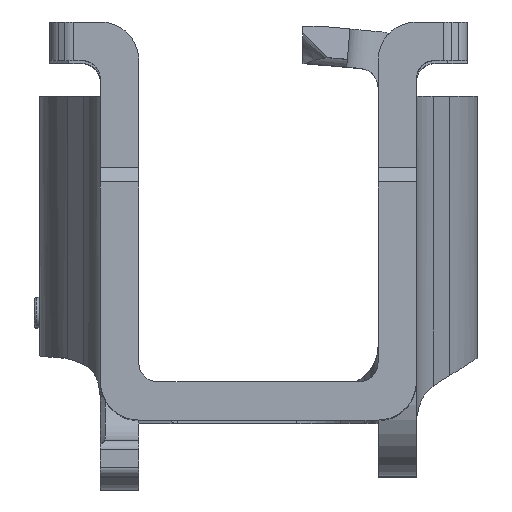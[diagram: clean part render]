
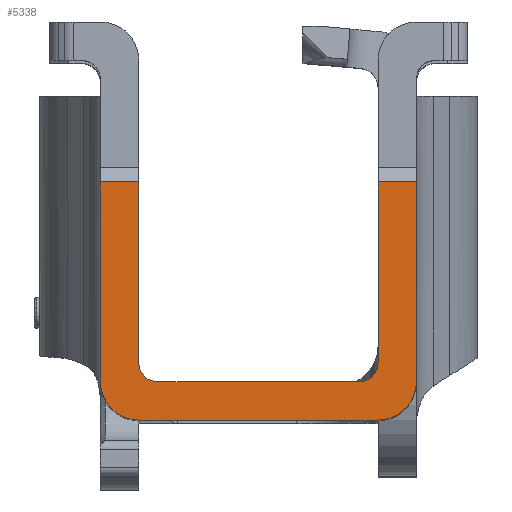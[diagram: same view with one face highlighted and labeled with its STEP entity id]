
A CAD part, top view. The second image highlights one B-rep face of the part: STEP entity #5338.
In plain terms, the highlighted planar face has unit normal (0, 0, 1).
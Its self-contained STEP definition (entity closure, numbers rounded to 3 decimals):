
#235=PLANE('',#5881);
#502=FACE_OUTER_BOUND('',#802,.T.);
#802=EDGE_LOOP('',(#4935,#4936,#4937,#4938,#4939,#4940,#4941,#4942,#4943,
#4944,#4945,#4946));
#888=LINE('',#7627,#1386);
#1201=LINE('',#8884,#1699);
#1208=LINE('',#8909,#1706);
#1216=LINE('',#8926,#1714);
#1217=LINE('',#8929,#1715);
#1227=LINE('',#8997,#1725);
#1259=LINE('',#9089,#1757);
#1299=LINE('',#9210,#1797);
#1386=VECTOR('',#6019,10.);
#1699=VECTOR('',#6978,10.);
#1706=VECTOR('',#7003,10.);
#1714=VECTOR('',#7017,10.);
#1715=VECTOR('',#7020,10.);
#1725=VECTOR('',#7068,10.);
#1757=VECTOR('',#7186,10.);
#1797=VECTOR('',#7322,10.);
#1920=CIRCLE('',#5492,1.);
#1921=CIRCLE('',#5494,1.);
#2044=CIRCLE('',#5830,2.);
#2045=CIRCLE('',#5838,2.);
#2107=VERTEX_POINT('',#7624);
#2108=VERTEX_POINT('',#7626);
#2239=VERTEX_POINT('',#7992);
#2240=VERTEX_POINT('',#7996);
#2241=VERTEX_POINT('',#7998);
#2506=VERTEX_POINT('',#8882);
#2514=VERTEX_POINT('',#8906);
#2515=VERTEX_POINT('',#8908);
#2522=VERTEX_POINT('',#8928);
#2535=VERTEX_POINT('',#8996);
#2568=VERTEX_POINT('',#9182);
#2569=VERTEX_POINT('',#9206);
#2647=EDGE_CURVE('',#2108,#2107,#888,.T.);
#2804=EDGE_CURVE('',#2239,#2107,#1920,.T.);
#2806=EDGE_CURVE('',#2240,#2241,#1921,.T.);
#3182=EDGE_CURVE('',#2240,#2506,#1201,.T.);
#3193=EDGE_CURVE('',#2515,#2514,#1208,.T.);
#3203=EDGE_CURVE('',#2506,#2515,#1216,.T.);
#3204=EDGE_CURVE('',#2522,#2108,#1217,.T.);
#3228=EDGE_CURVE('',#2535,#2522,#1227,.T.);
#3272=EDGE_CURVE('',#2239,#2241,#1259,.T.);
#3320=EDGE_CURVE('',#2568,#2514,#2044,.T.);
#3325=EDGE_CURVE('',#2535,#2569,#2045,.T.);
#3327=EDGE_CURVE('',#2568,#2569,#1299,.T.);
#4935=ORIENTED_EDGE('',*,*,#3204,.T.);
#4936=ORIENTED_EDGE('',*,*,#2647,.T.);
#4937=ORIENTED_EDGE('',*,*,#2804,.F.);
#4938=ORIENTED_EDGE('',*,*,#3272,.T.);
#4939=ORIENTED_EDGE('',*,*,#2806,.F.);
#4940=ORIENTED_EDGE('',*,*,#3182,.T.);
#4941=ORIENTED_EDGE('',*,*,#3203,.T.);
#4942=ORIENTED_EDGE('',*,*,#3193,.T.);
#4943=ORIENTED_EDGE('',*,*,#3320,.F.);
#4944=ORIENTED_EDGE('',*,*,#3327,.T.);
#4945=ORIENTED_EDGE('',*,*,#3325,.F.);
#4946=ORIENTED_EDGE('',*,*,#3228,.T.);
#5338=ADVANCED_FACE('',(#502),#235,.T.);
#5492=AXIS2_PLACEMENT_3D('',#7994,#6294,#6295);
#5494=AXIS2_PLACEMENT_3D('',#7999,#6299,#6300);
#5830=AXIS2_PLACEMENT_3D('',#9184,#7299,#7300);
#5838=AXIS2_PLACEMENT_3D('',#9207,#7317,#7318);
#5881=AXIS2_PLACEMENT_3D('',#9286,#7438,#7439);
#6019=DIRECTION('',(0.,-1.,0.));
#6294=DIRECTION('center_axis',(0.,0.,1.));
#6295=DIRECTION('ref_axis',(0.707,-0.707,0.));
#6299=DIRECTION('center_axis',(0.,0.,1.));
#6300=DIRECTION('ref_axis',(-0.707,-0.707,0.));
#6978=DIRECTION('',(0.,1.,0.));
#7003=DIRECTION('',(0.,-1.,0.));
#7017=DIRECTION('',(-1.,0.,0.));
#7020=DIRECTION('',(-1.,0.,0.));
#7068=DIRECTION('',(0.,1.,0.));
#7186=DIRECTION('',(-1.,0.,0.));
#7299=DIRECTION('center_axis',(0.,0.,-1.));
#7300=DIRECTION('ref_axis',(-0.707,-0.707,0.));
#7317=DIRECTION('center_axis',(0.,0.,-1.));
#7318=DIRECTION('ref_axis',(0.707,-0.707,0.));
#7322=DIRECTION('',(1.,0.,0.));
#7438=DIRECTION('center_axis',(0.,0.,1.));
#7439=DIRECTION('ref_axis',(1.,0.,0.));
#7624=CARTESIAN_POINT('',(6.25,-15.8,110.25));
#7626=CARTESIAN_POINT('',(6.25,-6.36,110.25));
#7627=CARTESIAN_POINT('',(6.25,-1.81,110.25));
#7992=CARTESIAN_POINT('',(5.25,-16.8,110.25));
#7994=CARTESIAN_POINT('Origin',(5.25,-15.8,110.25));
#7996=CARTESIAN_POINT('',(-6.25,-15.8,110.25));
#7998=CARTESIAN_POINT('',(-5.25,-16.8,110.25));
#7999=CARTESIAN_POINT('Origin',(-5.25,-15.8,110.25));
#8882=CARTESIAN_POINT('',(-6.25,-6.36,110.25));
#8884=CARTESIAN_POINT('',(-6.25,-16.8,110.25));
#8906=CARTESIAN_POINT('',(-8.25,-16.8,110.25));
#8908=CARTESIAN_POINT('',(-8.25,-6.36,110.25));
#8909=CARTESIAN_POINT('',(-8.25,-1.81,110.25));
#8926=CARTESIAN_POINT('',(4.125,-6.36,110.25));
#8928=CARTESIAN_POINT('',(8.25,-6.36,110.25));
#8929=CARTESIAN_POINT('',(4.125,-6.36,110.25));
#8996=CARTESIAN_POINT('',(8.25,-16.8,110.25));
#8997=CARTESIAN_POINT('',(8.25,-18.8,110.25));
#9089=CARTESIAN_POINT('',(6.25,-16.8,110.25));
#9182=CARTESIAN_POINT('',(-6.25,-18.8,110.25));
#9184=CARTESIAN_POINT('Origin',(-6.25,-16.8,110.25));
#9206=CARTESIAN_POINT('',(6.25,-18.8,110.25));
#9207=CARTESIAN_POINT('Origin',(6.25,-16.8,110.25));
#9210=CARTESIAN_POINT('',(-8.25,-18.8,110.25));
#9286=CARTESIAN_POINT('Origin',(0.,-10.305,110.25));
